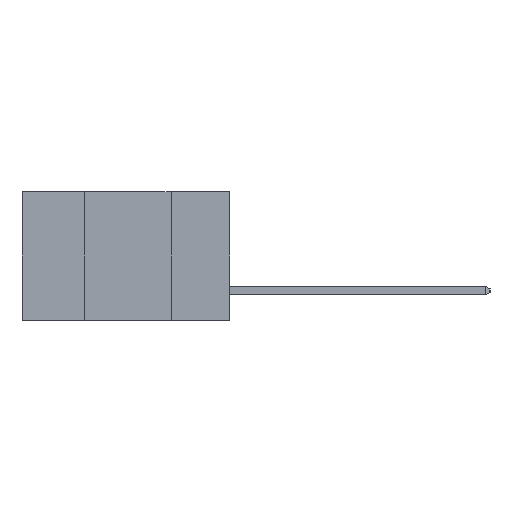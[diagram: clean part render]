
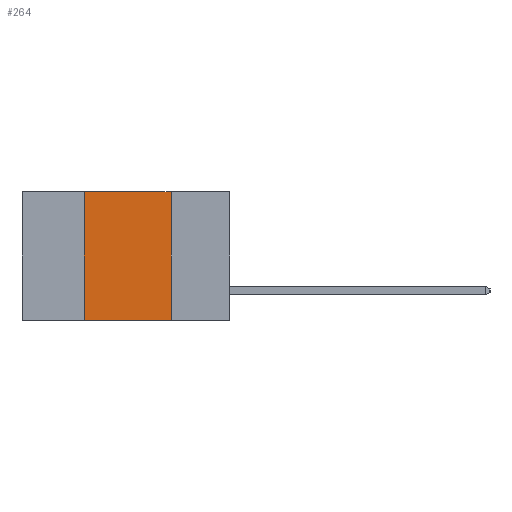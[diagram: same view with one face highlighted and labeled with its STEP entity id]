
A CAD part, left-side view. The second image highlights one B-rep face of the part: STEP entity #264.
In plain terms, the highlighted planar face has unit normal (-1, 0, 0).
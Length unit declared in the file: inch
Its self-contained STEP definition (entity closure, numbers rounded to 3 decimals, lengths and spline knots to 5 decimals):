
#264 = ADVANCED_FACE ( 'NONE', ( #21177 ), #18917, .F. ) ;
#471 = AXIS2_PLACEMENT_3D ( 'NONE', #18337, #18841, #18760 ) ;
#2749 = EDGE_CURVE ( 'NONE', #13755, #15411, #13868, .T. ) ;
#2754 = ORIENTED_EDGE ( 'NONE', *, *, #3947, .F. ) ;
#3947 = EDGE_CURVE ( 'NONE', #16671, #15411, #23254, .T. ) ;
#7887 = CARTESIAN_POINT ( 'NONE',  ( 0., 0.6, 0. ) ) ;
#8595 = EDGE_CURVE ( 'NONE', #15061, #16671, #15872, .T. ) ;
#8830 = ORIENTED_EDGE ( 'NONE', *, *, #2749, .T. ) ;
#11783 = VECTOR ( 'NONE', #13863, 39.37008 ) ;
#12427 = VECTOR ( 'NONE', #21271, 39.37008 ) ;
#13184 = ORIENTED_EDGE ( 'NONE', *, *, #8595, .F. ) ;
#13547 = CARTESIAN_POINT ( 'NONE',  ( 0., 0.17, 0. ) ) ;
#13755 = VERTEX_POINT ( 'NONE', #21796 ) ;
#13863 = DIRECTION ( 'NONE',  ( 0., 0., -1. ) ) ;
#13868 = LINE ( 'NONE', #18397, #18217 ) ;
#15061 = VERTEX_POINT ( 'NONE', #20664 ) ;
#15411 = VERTEX_POINT ( 'NONE', #16124 ) ;
#15872 = LINE ( 'NONE', #7887, #20196 ) ;
#16124 = CARTESIAN_POINT ( 'NONE',  ( 0., 0.17, -0.37 ) ) ;
#16671 = VERTEX_POINT ( 'NONE', #20831 ) ;
#17120 = DIRECTION ( 'NONE',  ( 0., -1., 0. ) ) ;
#18217 = VECTOR ( 'NONE', #22736, 39.37008 ) ;
#18337 = CARTESIAN_POINT ( 'NONE',  ( 0., 0.6, 0. ) ) ;
#18397 = CARTESIAN_POINT ( 'NONE',  ( 0., 0.6, -0.37 ) ) ;
#18760 = DIRECTION ( 'NONE',  ( 0., 0., -1. ) ) ;
#18841 = DIRECTION ( 'NONE',  ( 1., 0., 0. ) ) ;
#18917 = PLANE ( 'NONE',  #471 ) ;
#19438 = CARTESIAN_POINT ( 'NONE',  ( 0., 0.42, 0. ) ) ;
#20196 = VECTOR ( 'NONE', #17120, 39.37008 ) ;
#20664 = CARTESIAN_POINT ( 'NONE',  ( 0., 0.42, 0. ) ) ;
#20831 = CARTESIAN_POINT ( 'NONE',  ( 0., 0.17, 0. ) ) ;
#20832 = EDGE_LOOP ( 'NONE', ( #2754, #13184, #22931, #8830 ) ) ;
#21177 = FACE_OUTER_BOUND ( 'NONE', #20832, .T. ) ;
#21271 = DIRECTION ( 'NONE',  ( 0., 0., 1. ) ) ;
#21796 = CARTESIAN_POINT ( 'NONE',  ( 0., 0.42, -0.37 ) ) ;
#22193 = LINE ( 'NONE', #19438, #12427 ) ;
#22736 = DIRECTION ( 'NONE',  ( 0., -1., 0. ) ) ;
#22793 = EDGE_CURVE ( 'NONE', #13755, #15061, #22193, .T. ) ;
#22931 = ORIENTED_EDGE ( 'NONE', *, *, #22793, .F. ) ;
#23254 = LINE ( 'NONE', #13547, #11783 ) ;
